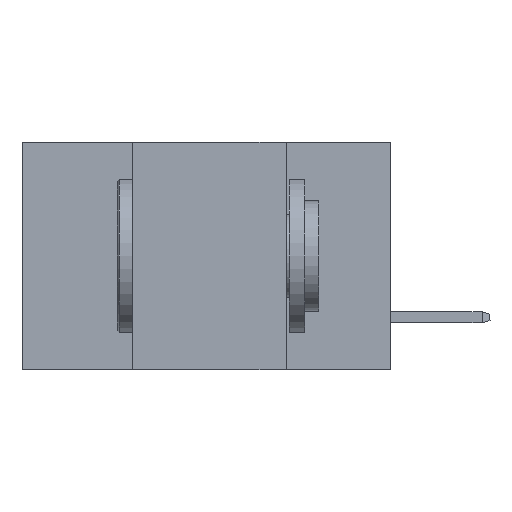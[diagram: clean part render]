
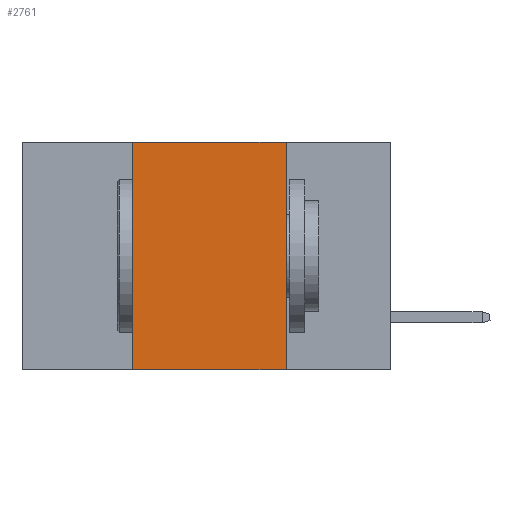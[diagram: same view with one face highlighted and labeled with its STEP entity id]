
A CAD part, left-side view. The second image highlights one B-rep face of the part: STEP entity #2761.
In plain terms, the highlighted planar face has unit normal (-1, 0, 0).
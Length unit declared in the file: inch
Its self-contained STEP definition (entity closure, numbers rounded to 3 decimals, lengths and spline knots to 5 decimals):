
#1175 = FACE_OUTER_BOUND ( 'NONE', #16752, .T. ) ;
#2278 = LINE ( 'NONE', #22923, #22175 ) ;
#2761 = ADVANCED_FACE ( 'NONE', ( #1175 ), #8545, .F. ) ;
#3334 = CARTESIAN_POINT ( 'NONE',  ( 0., 0.17, 0. ) ) ;
#3400 = LINE ( 'NONE', #21701, #24438 ) ;
#4149 = ORIENTED_EDGE ( 'NONE', *, *, #16982, .T. ) ;
#4701 = LINE ( 'NONE', #19910, #25084 ) ;
#5568 = LINE ( 'NONE', #3334, #20804 ) ;
#7125 = DIRECTION ( 'NONE',  ( 0., 0., 1. ) ) ;
#8271 = ORIENTED_EDGE ( 'NONE', *, *, #13871, .F. ) ;
#8437 = DIRECTION ( 'NONE',  ( 0., 0., -1. ) ) ;
#8464 = DIRECTION ( 'NONE',  ( 1., 0., 0. ) ) ;
#8545 = PLANE ( 'NONE',  #18808 ) ;
#8796 = CARTESIAN_POINT ( 'NONE',  ( 0., 0.6, 0. ) ) ;
#10987 = CARTESIAN_POINT ( 'NONE',  ( 0., 0.17, 0. ) ) ;
#11394 = CARTESIAN_POINT ( 'NONE',  ( 0., 0.42, -0.37 ) ) ;
#11416 = DIRECTION ( 'NONE',  ( 0., 0., -1. ) ) ;
#12347 = ORIENTED_EDGE ( 'NONE', *, *, #19551, .F. ) ;
#12991 = CARTESIAN_POINT ( 'NONE',  ( 0., 0.17, -0.37 ) ) ;
#13871 = EDGE_CURVE ( 'NONE', #14976, #24134, #2278, .T. ) ;
#14976 = VERTEX_POINT ( 'NONE', #11394 ) ;
#15993 = DIRECTION ( 'NONE',  ( 0., -1., 0. ) ) ;
#16752 = EDGE_LOOP ( 'NONE', ( #12347, #23371, #8271, #4149 ) ) ;
#16982 = EDGE_CURVE ( 'NONE', #14976, #21733, #3400, .T. ) ;
#18808 = AXIS2_PLACEMENT_3D ( 'NONE', #8796, #8464, #8437 ) ;
#18900 = CARTESIAN_POINT ( 'NONE',  ( 0., 0.42, 0. ) ) ;
#19551 = EDGE_CURVE ( 'NONE', #21128, #21733, #5568, .T. ) ;
#19910 = CARTESIAN_POINT ( 'NONE',  ( 0., 0.6, 0. ) ) ;
#20804 = VECTOR ( 'NONE', #11416, 39.37008 ) ;
#21128 = VERTEX_POINT ( 'NONE', #10987 ) ;
#21701 = CARTESIAN_POINT ( 'NONE',  ( 0., 0.6, -0.37 ) ) ;
#21733 = VERTEX_POINT ( 'NONE', #12991 ) ;
#22175 = VECTOR ( 'NONE', #7125, 39.37008 ) ;
#22923 = CARTESIAN_POINT ( 'NONE',  ( 0., 0.42, 0. ) ) ;
#23371 = ORIENTED_EDGE ( 'NONE', *, *, #23824, .F. ) ;
#23824 = EDGE_CURVE ( 'NONE', #24134, #21128, #4701, .T. ) ;
#24134 = VERTEX_POINT ( 'NONE', #18900 ) ;
#24438 = VECTOR ( 'NONE', #25539, 39.37008 ) ;
#25084 = VECTOR ( 'NONE', #15993, 39.37008 ) ;
#25539 = DIRECTION ( 'NONE',  ( 0., -1., 0. ) ) ;
